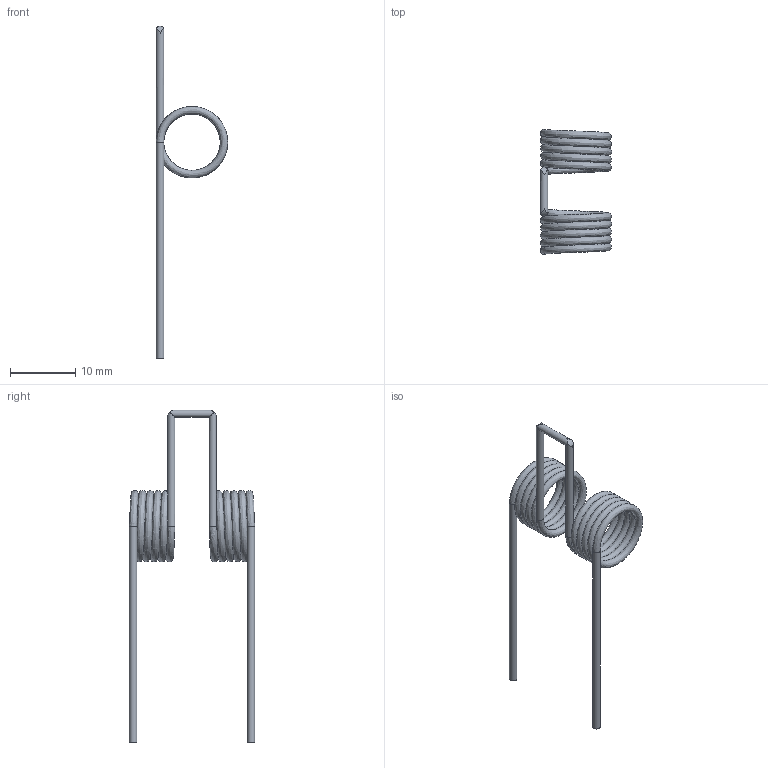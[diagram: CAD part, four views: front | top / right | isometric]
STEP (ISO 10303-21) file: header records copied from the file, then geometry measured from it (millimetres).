
FILE_DESCRIPTION(/* description */ (''),/* implementation_level */ '2;1');
FILE_NAME(/* name */ 'Hammer Spring.stp',/* time_stamp */ '2018-09-18T03:18:38-05:00',/* author */ ('johne'),/* organization */ (''),/* preprocessor_version */ 'ST-DEVELOPER v16.13',/* originating_system */ 'Autodesk Inventor 2018',/* authorisation */ '');
FILE_SCHEMA (('AUTOMOTIVE_DESIGN { 1 0 10303 214 3 1 1 }'));
Length unit declared in the file: inch
Products named in the file (1): Hammer Spring
Bounding box: 10.92 x 19.18 x 50.8 mm (x, y, z)
Volume: 424.5 mm3; surface area: 1487.1 mm2
Topology: 1 solids, 1 shells, 11 faces, 35 edges, 26 vertices
Faces by surface type: cylinder 7, plane 2, bspline 2
Full cylindrical faces by diameter (mm): 1.143 x5
Entity records: 2257 total; most frequent: CARTESIAN_POINT 1918, ORIENTED_EDGE 60, DIRECTION 52, EDGE_CURVE 30, VERTEX_POINT 26, AXIS2_PLACEMENT_3D 26, EDGE_LOOP 24, B_SPLINE_CURVE_WITH_KNOTS 14
